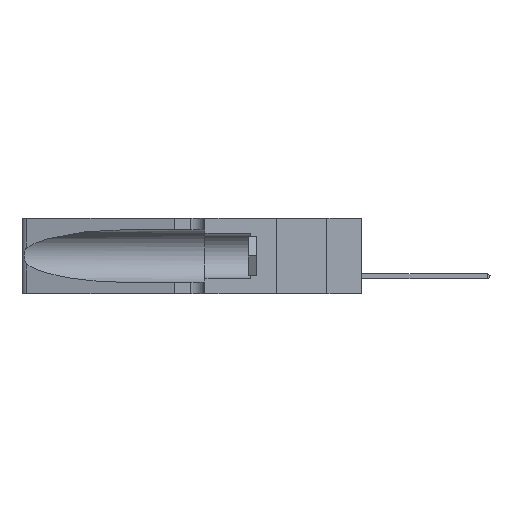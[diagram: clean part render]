
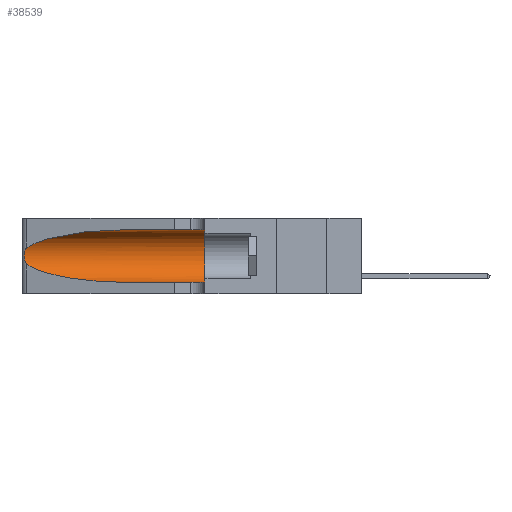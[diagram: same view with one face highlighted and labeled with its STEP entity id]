
A CAD part, left-side view. The second image highlights one B-rep face of the part: STEP entity #38539.
In plain terms, the highlighted cylindrical face has radius 3.308 mm (diameter 6.617 mm), a partial arc.
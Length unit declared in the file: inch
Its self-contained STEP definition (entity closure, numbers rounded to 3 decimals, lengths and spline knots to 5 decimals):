
#46 = VERTEX_POINT ( 'NONE', #42409 ) ;
#647 = DIRECTION ( 'NONE',  ( 0., 0., -1. ) ) ;
#692 = CARTESIAN_POINT ( 'NONE',  ( 0.1305, 1.61858, 0.31525 ) ) ;
#3446 = CARTESIAN_POINT ( 'NONE',  ( 0.2373, 1.15595, 0.28018 ) ) ;
#3464 = VECTOR ( 'NONE', #6310, 39.37008 ) ;
#3594 =( BOUNDED_CURVE ( )  B_SPLINE_CURVE ( 3, ( #31681, #41650, #35182, #21271 ),
 .UNSPECIFIED., .F., .T. ) 
 B_SPLINE_CURVE_WITH_KNOTS ( ( 4, 4 ),
 ( 3.44316, 4.71239 ),
 .UNSPECIFIED. ) 
 CURVE ( )  GEOMETRIC_REPRESENTATION_ITEM ( )  RATIONAL_B_SPLINE_CURVE ( ( 1., 0.87, 0.87, 1. ) ) 
 REPRESENTATION_ITEM ( '' )  );
#3598 = CARTESIAN_POINT ( 'NONE',  ( 0.25487, 1.22718, 0.22369 ) ) ;
#5061 = CARTESIAN_POINT ( 'NONE',  ( 0.25487, 1.22718, 0.22369 ) ) ;
#6204 = AXIS2_PLACEMENT_3D ( 'NONE', #26305, #36804, #43565 ) ;
#6310 = DIRECTION ( 'NONE',  ( 0., -1., 0. ) ) ;
#6563 = CARTESIAN_POINT ( 'NONE',  ( 0.26075, 1.23896, 0.19203 ) ) ;
#10164 = CARTESIAN_POINT ( 'NONE',  ( 0.26018, 1.23835, 0.19895 ) ) ;
#10593 = CARTESIAN_POINT ( 'NONE',  ( 0.25854, 1.2359, 0.20912 ) ) ;
#11046 = VERTEX_POINT ( 'NONE', #34618 ) ;
#11908 = VERTEX_POINT ( 'NONE', #5061 ) ;
#12687 = EDGE_CURVE ( 'NONE', #11908, #34427, #35392, .T. ) ;
#12688 = LINE ( 'NONE', #20108, #3464 ) ;
#12918 = VERTEX_POINT ( 'NONE', #35587 ) ;
#14543 = CARTESIAN_POINT ( 'NONE',  ( 0.25555, 1.22993, 0.14849 ) ) ;
#16134 = CARTESIAN_POINT ( 'NONE',  ( 0.25487, 1.22718, 0.14631 ) ) ;
#17101 = ORIENTED_EDGE ( 'NONE', *, *, #23313, .T. ) ;
#17312 = CARTESIAN_POINT ( 'NONE',  ( 0.26017, 1.23833, 0.17102 ) ) ;
#17445 = CARTESIAN_POINT ( 'NONE',  ( 0.25787, 1.23484, 0.2124 ) ) ;
#18218 = CARTESIAN_POINT ( 'NONE',  ( 0.25487, 1.22718, 0.14631 ) ) ;
#20066 = CARTESIAN_POINT ( 'NONE',  ( 0.25555, 1.22994, 0.2215 ) ) ;
#20108 = CARTESIAN_POINT ( 'NONE',  ( 0.1305, 1.61858, 0.05475 ) ) ;
#20209 = CARTESIAN_POINT ( 'NONE',  ( 0.25487, 1.22718, 0.22369 ) ) ;
#20210 = EDGE_CURVE ( 'NONE', #34427, #46, #3594, .T. ) ;
#21271 = CARTESIAN_POINT ( 'NONE',  ( 0.1305, 0.72297, 0.05475 ) ) ;
#21498 = DIRECTION ( 'NONE',  ( 0., -1., 0. ) ) ;
#22077 = VECTOR ( 'NONE', #25391, 39.37008 ) ;
#22096 = EDGE_CURVE ( 'NONE', #11046, #12918, #40567, .T. ) ;
#23313 = EDGE_CURVE ( 'NONE', #46, #32215, #12688, .T. ) ;
#24246 = EDGE_CURVE ( 'NONE', #11046, #11908, #42015, .T. ) ;
#24438 = CARTESIAN_POINT ( 'NONE',  ( 0.18966, 0.96281, 0.31525 ) ) ;
#25188 = EDGE_CURVE ( 'NONE', #12918, #32215, #39211, .T. ) ;
#25391 = DIRECTION ( 'NONE',  ( 0., -1., 0. ) ) ;
#26045 = ORIENTED_EDGE ( 'NONE', *, *, #24246, .T. ) ;
#26305 = CARTESIAN_POINT ( 'NONE',  ( 0.1305, 0.35, 0.185 ) ) ;
#27260 = CARTESIAN_POINT ( 'NONE',  ( 0.25639, 1.23184, 0.21858 ) ) ;
#27739 = AXIS2_PLACEMENT_3D ( 'NONE', #42299, #21498, #647 ) ;
#28583 = CARTESIAN_POINT ( 'NONE',  ( 0.25639, 1.23186, 0.15144 ) ) ;
#31646 = CARTESIAN_POINT ( 'NONE',  ( 0.25789, 1.23486, 0.15765 ) ) ;
#31681 = CARTESIAN_POINT ( 'NONE',  ( 0.25487, 1.22718, 0.14631 ) ) ;
#31739 = FACE_OUTER_BOUND ( 'NONE', #36859, .T. ) ;
#32215 = VERTEX_POINT ( 'NONE', #42194 ) ;
#33382 = CYLINDRICAL_SURFACE ( 'NONE', #27739, 0.13025 ) ;
#33474 = ORIENTED_EDGE ( 'NONE', *, *, #25188, .F. ) ;
#34427 = VERTEX_POINT ( 'NONE', #16134 ) ;
#34567 = CARTESIAN_POINT ( 'NONE',  ( 0.26075, 1.23896, 0.178 ) ) ;
#34618 = CARTESIAN_POINT ( 'NONE',  ( 0.1305, 0.72297, 0.31525 ) ) ;
#35182 = CARTESIAN_POINT ( 'NONE',  ( 0.18966, 0.96281, 0.05475 ) ) ;
#35392 = B_SPLINE_CURVE_WITH_KNOTS ( 'NONE', 3,
 ( #20209, #20066, #27260, #17445, #10593, #10164, #6563, #34567, #17312, #39023, #31646, #28583, #14543, #18218 ),
 .UNSPECIFIED., .F., .F.,
 ( 4, 2, 2, 2, 2, 2, 4 ),
 ( 0., 0.00027, 0.00053, 0.00107, 0.0016, 0.00187, 0.00214 ),
 .UNSPECIFIED. ) ;
#35587 = CARTESIAN_POINT ( 'NONE',  ( 0.1305, 0.35, 0.31525 ) ) ;
#36804 = DIRECTION ( 'NONE',  ( 0., 1., 0. ) ) ;
#36859 = EDGE_LOOP ( 'NONE', ( #26045, #44658, #38402, #17101, #33474, #44621 ) ) ;
#38402 = ORIENTED_EDGE ( 'NONE', *, *, #20210, .T. ) ;
#38539 = ADVANCED_FACE ( 'NONE', ( #31739 ), #33382, .F. ) ;
#39023 = CARTESIAN_POINT ( 'NONE',  ( 0.25856, 1.23593, 0.16098 ) ) ;
#39211 = CIRCLE ( 'NONE', #6204, 0.13025 ) ;
#40567 = LINE ( 'NONE', #692, #22077 ) ;
#41650 = CARTESIAN_POINT ( 'NONE',  ( 0.2373, 1.15595, 0.08982 ) ) ;
#42015 =( BOUNDED_CURVE ( )  B_SPLINE_CURVE ( 3, ( #42305, #24438, #3446, #3598 ),
 .UNSPECIFIED., .F., .F. ) 
 B_SPLINE_CURVE_WITH_KNOTS ( ( 4, 4 ),
 ( 1.5708, 2.84003 ),
 .UNSPECIFIED. ) 
 CURVE ( )  GEOMETRIC_REPRESENTATION_ITEM ( )  RATIONAL_B_SPLINE_CURVE ( ( 1., 0.87, 0.87, 1. ) ) 
 REPRESENTATION_ITEM ( '' )  );
#42194 = CARTESIAN_POINT ( 'NONE',  ( 0.1305, 0.35, 0.05475 ) ) ;
#42299 = CARTESIAN_POINT ( 'NONE',  ( 0.1305, 1.61858, 0.185 ) ) ;
#42305 = CARTESIAN_POINT ( 'NONE',  ( 0.1305, 0.72297, 0.31525 ) ) ;
#42409 = CARTESIAN_POINT ( 'NONE',  ( 0.1305, 0.72297, 0.05475 ) ) ;
#43565 = DIRECTION ( 'NONE',  ( 0., 0., 1. ) ) ;
#44621 = ORIENTED_EDGE ( 'NONE', *, *, #22096, .F. ) ;
#44658 = ORIENTED_EDGE ( 'NONE', *, *, #12687, .T. ) ;
